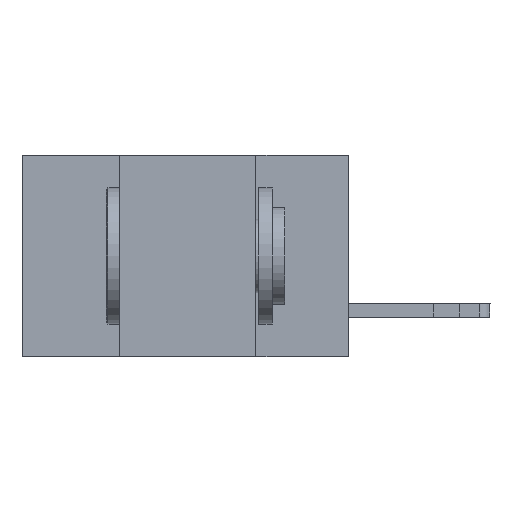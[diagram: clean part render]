
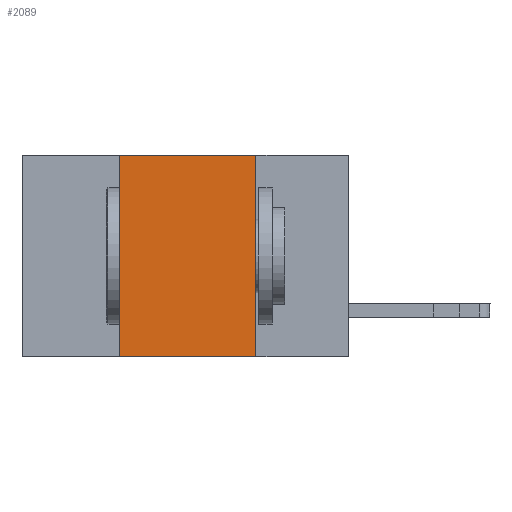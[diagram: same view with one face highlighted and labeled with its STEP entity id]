
A CAD part, left-side view. The second image highlights one B-rep face of the part: STEP entity #2089.
In plain terms, the highlighted planar face has unit normal (-1, 0, 0).
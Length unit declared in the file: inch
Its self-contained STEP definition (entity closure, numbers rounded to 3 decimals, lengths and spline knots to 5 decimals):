
#119 = EDGE_CURVE ( 'NONE', #1036, #3148, #6965, .T. ) ;
#187 = DIRECTION ( 'NONE',  ( 1., 0., 0. ) ) ;
#225 = DIRECTION ( 'NONE',  ( 0., -1., 0. ) ) ;
#266 = DIRECTION ( 'NONE',  ( 0., -1., 0. ) ) ;
#734 = AXIS2_PLACEMENT_3D ( 'NONE', #3789, #187, #8067 ) ;
#1029 = LINE ( 'NONE', #9175, #6112 ) ;
#1036 = VERTEX_POINT ( 'NONE', #8759 ) ;
#1049 = LINE ( 'NONE', #4587, #4785 ) ;
#1298 = VECTOR ( 'NONE', #5313, 39.37008 ) ;
#1302 = VERTEX_POINT ( 'NONE', #3961 ) ;
#1337 = CARTESIAN_POINT ( 'NONE',  ( 0., 0.42, -0.37 ) ) ;
#1634 = EDGE_CURVE ( 'NONE', #10767, #1302, #1049, .T. ) ;
#2089 = ADVANCED_FACE ( 'NONE', ( #11288 ), #8558, .F. ) ;
#2639 = EDGE_CURVE ( 'NONE', #10767, #3148, #1029, .T. ) ;
#2942 = CARTESIAN_POINT ( 'NONE',  ( 0., 0.17, -0.37 ) ) ;
#3099 = ORIENTED_EDGE ( 'NONE', *, *, #119, .F. ) ;
#3148 = VERTEX_POINT ( 'NONE', #2942 ) ;
#3789 = CARTESIAN_POINT ( 'NONE',  ( 0., 0.6, 0. ) ) ;
#3961 = CARTESIAN_POINT ( 'NONE',  ( 0., 0.42, 0. ) ) ;
#4587 = CARTESIAN_POINT ( 'NONE',  ( 0., 0.42, -0.37 ) ) ;
#4785 = VECTOR ( 'NONE', #8653, 39.37008 ) ;
#5142 = ORIENTED_EDGE ( 'NONE', *, *, #2639, .T. ) ;
#5313 = DIRECTION ( 'NONE',  ( 0., 0., -1. ) ) ;
#5536 = EDGE_LOOP ( 'NONE', ( #3099, #6144, #6676, #5142 ) ) ;
#6112 = VECTOR ( 'NONE', #225, 39.37008 ) ;
#6144 = ORIENTED_EDGE ( 'NONE', *, *, #9774, .F. ) ;
#6676 = ORIENTED_EDGE ( 'NONE', *, *, #1634, .F. ) ;
#6965 = LINE ( 'NONE', #8002, #1298 ) ;
#8002 = CARTESIAN_POINT ( 'NONE',  ( 0., 0.17, -0.37 ) ) ;
#8067 = DIRECTION ( 'NONE',  ( 0., 0., -1. ) ) ;
#8222 = CARTESIAN_POINT ( 'NONE',  ( 0., 0.6, 0. ) ) ;
#8558 = PLANE ( 'NONE',  #734 ) ;
#8653 = DIRECTION ( 'NONE',  ( 0., 0., 1. ) ) ;
#8759 = CARTESIAN_POINT ( 'NONE',  ( 0., 0.17, 0. ) ) ;
#9175 = CARTESIAN_POINT ( 'NONE',  ( 0., 0.6, -0.37 ) ) ;
#9774 = EDGE_CURVE ( 'NONE', #1302, #1036, #9842, .T. ) ;
#9842 = LINE ( 'NONE', #8222, #10673 ) ;
#10673 = VECTOR ( 'NONE', #266, 39.37008 ) ;
#10767 = VERTEX_POINT ( 'NONE', #1337 ) ;
#11288 = FACE_OUTER_BOUND ( 'NONE', #5536, .T. ) ;
